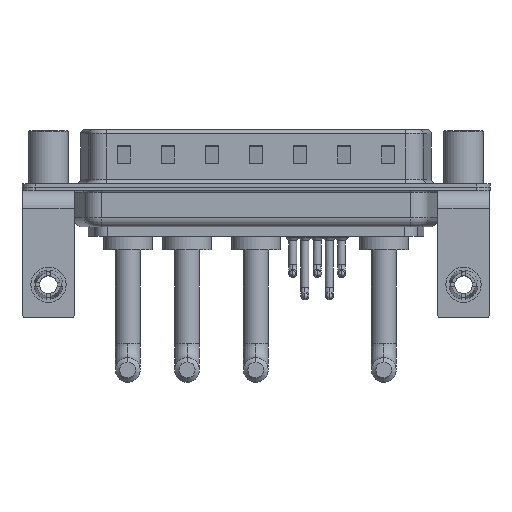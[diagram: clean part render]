
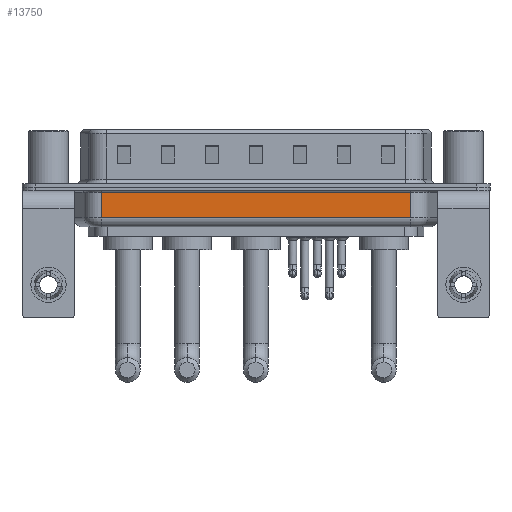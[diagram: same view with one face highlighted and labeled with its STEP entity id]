
A CAD part, front view. The second image highlights one B-rep face of the part: STEP entity #13750.
In plain terms, the highlighted planar face has unit normal (0, -1, 0).
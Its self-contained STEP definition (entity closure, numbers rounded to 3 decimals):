
#865 = DIRECTION ( 'NONE',  ( 0., 0., 1. ) ) ;
#1631 = DIRECTION ( 'NONE',  ( 0., 0., 1. ) ) ;
#1632 = LINE ( 'NONE', #17256, #8993 ) ;
#2045 = DIRECTION ( 'NONE',  ( 1., 0., 0. ) ) ;
#3121 = DIRECTION ( 'NONE',  ( 0., 0., 1. ) ) ;
#3916 = CARTESIAN_POINT ( 'NONE',  ( 6.006, -5.35, -4.5 ) ) ;
#4068 = DIRECTION ( 'NONE',  ( -1., 0., 0. ) ) ;
#4413 = ORIENTED_EDGE ( 'NONE', *, *, #8078, .T. ) ;
#5112 = VECTOR ( 'NONE', #2045, 1000. ) ;
#5260 = FACE_OUTER_BOUND ( 'NONE', #26530, .T. ) ;
#7371 = EDGE_CURVE ( 'NONE', #14030, #17866, #18572, .T. ) ;
#7597 = CARTESIAN_POINT ( 'NONE',  ( 6.006, -5.35, -0.65 ) ) ;
#8078 = EDGE_CURVE ( 'NONE', #17866, #14352, #1632, .T. ) ;
#8808 = VECTOR ( 'NONE', #1631, 1000. ) ;
#8993 = VECTOR ( 'NONE', #865, 1000. ) ;
#9195 = VERTEX_POINT ( 'NONE', #7597 ) ;
#10281 = ORIENTED_EDGE ( 'NONE', *, *, #26356, .F. ) ;
#12128 = LINE ( 'NONE', #24112, #16536 ) ;
#13750 = ADVANCED_FACE ( 'NONE', ( #5260 ), #15093, .F. ) ;
#14030 = VERTEX_POINT ( 'NONE', #24869 ) ;
#14352 = VERTEX_POINT ( 'NONE', #21759 ) ;
#15093 = PLANE ( 'NONE',  #21098 ) ;
#16536 = VECTOR ( 'NONE', #4068, 1000. ) ;
#16551 = CARTESIAN_POINT ( 'NONE',  ( 6.006, -5.35, -3.5 ) ) ;
#17256 = CARTESIAN_POINT ( 'NONE',  ( 41.044, -5.35, -4.5 ) ) ;
#17866 = VERTEX_POINT ( 'NONE', #26357 ) ;
#18572 = LINE ( 'NONE', #16551, #5112 ) ;
#18681 = ORIENTED_EDGE ( 'NONE', *, *, #21561, .T. ) ;
#21098 = AXIS2_PLACEMENT_3D ( 'NONE', #21550, #21687, #3121 ) ;
#21550 = CARTESIAN_POINT ( 'NONE',  ( 6.006, -5.35, -4.5 ) ) ;
#21561 = EDGE_CURVE ( 'NONE', #14352, #9195, #12128, .T. ) ;
#21687 = DIRECTION ( 'NONE',  ( 0., 1., 0. ) ) ;
#21759 = CARTESIAN_POINT ( 'NONE',  ( 41.044, -5.35, -0.65 ) ) ;
#24112 = CARTESIAN_POINT ( 'NONE',  ( 6.006, -5.35, -0.65 ) ) ;
#24624 = LINE ( 'NONE', #3916, #8808 ) ;
#24869 = CARTESIAN_POINT ( 'NONE',  ( 6.006, -5.35, -3.5 ) ) ;
#25449 = ORIENTED_EDGE ( 'NONE', *, *, #7371, .T. ) ;
#26356 = EDGE_CURVE ( 'NONE', #14030, #9195, #24624, .T. ) ;
#26357 = CARTESIAN_POINT ( 'NONE',  ( 41.044, -5.35, -3.5 ) ) ;
#26530 = EDGE_LOOP ( 'NONE', ( #10281, #25449, #4413, #18681 ) ) ;
